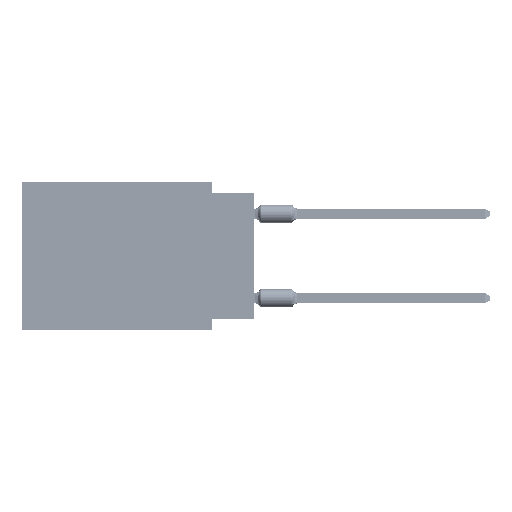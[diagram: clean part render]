
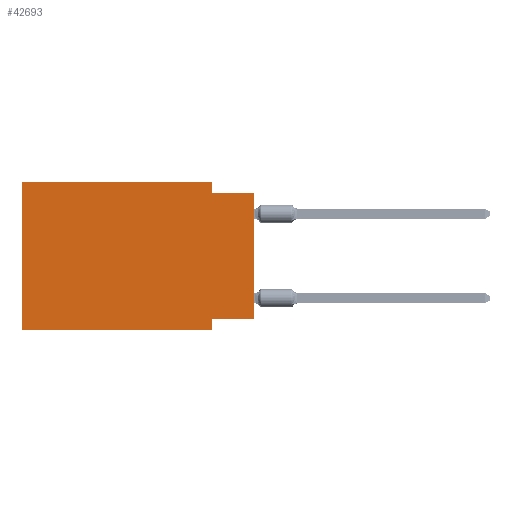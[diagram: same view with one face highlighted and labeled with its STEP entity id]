
A CAD part, left-side view. The second image highlights one B-rep face of the part: STEP entity #42693.
In plain terms, the highlighted planar face has unit normal (-1, 0, 0).
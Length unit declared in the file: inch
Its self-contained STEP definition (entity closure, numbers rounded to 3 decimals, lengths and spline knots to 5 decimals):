
#1951 = EDGE_CURVE ( 'NONE', #13070, #85493, #46114, .T. ) ;
#2984 = VECTOR ( 'NONE', #79374, 39.37008 ) ;
#6643 = DIRECTION ( 'NONE',  ( 0., 0., -1. ) ) ;
#12894 = LINE ( 'NONE', #95764, #94227 ) ;
#13070 = VERTEX_POINT ( 'NONE', #76382 ) ;
#13754 = VERTEX_POINT ( 'NONE', #31894 ) ;
#15573 = EDGE_CURVE ( 'NONE', #13754, #57237, #38477, .T. ) ;
#16626 = ORIENTED_EDGE ( 'NONE', *, *, #24717, .F. ) ;
#17068 = VECTOR ( 'NONE', #44980, 39.37008 ) ;
#18312 = CARTESIAN_POINT ( 'NONE',  ( 0., 0.55, 0. ) ) ;
#18451 = EDGE_LOOP ( 'NONE', ( #107226, #99488, #53369, #82596, #94950, #79710, #16626, #52889 ) ) ;
#20649 = CARTESIAN_POINT ( 'NONE',  ( 0., 0., 0. ) ) ;
#21079 = DIRECTION ( 'NONE',  ( 0., 0., -1. ) ) ;
#23228 = AXIS2_PLACEMENT_3D ( 'NONE', #80891, #97754, #73250 ) ;
#24717 = EDGE_CURVE ( 'NONE', #39532, #85493, #71554, .T. ) ;
#27841 = VECTOR ( 'NONE', #30315, 39.37008 ) ;
#30103 = VERTEX_POINT ( 'NONE', #82910 ) ;
#30315 = DIRECTION ( 'NONE',  ( 0., 0., 1. ) ) ;
#30742 = LINE ( 'NONE', #63977, #17068 ) ;
#31894 = CARTESIAN_POINT ( 'NONE',  ( 0., 0.1, -0.025 ) ) ;
#32446 = CARTESIAN_POINT ( 'NONE',  ( 0., 0.55, 0. ) ) ;
#36902 = LINE ( 'NONE', #86508, #27841 ) ;
#38477 = LINE ( 'NONE', #103917, #2984 ) ;
#39463 = PLANE ( 'NONE',  #23228 ) ;
#39532 = VERTEX_POINT ( 'NONE', #76016 ) ;
#42693 = ADVANCED_FACE ( 'NONE', ( #46021 ), #39463, .F. ) ;
#44980 = DIRECTION ( 'NONE',  ( 0., 1., 0. ) ) ;
#46021 = FACE_OUTER_BOUND ( 'NONE', #18451, .T. ) ;
#46114 = LINE ( 'NONE', #80439, #86129 ) ;
#49419 = VECTOR ( 'NONE', #6643, 39.37008 ) ;
#52889 = ORIENTED_EDGE ( 'NONE', *, *, #91686, .F. ) ;
#53369 = ORIENTED_EDGE ( 'NONE', *, *, #80028, .F. ) ;
#53909 = DIRECTION ( 'NONE',  ( 0., 0., 1. ) ) ;
#55893 = DIRECTION ( 'NONE',  ( 0., -1., 0. ) ) ;
#56287 = VECTOR ( 'NONE', #84206, 39.37008 ) ;
#57237 = VERTEX_POINT ( 'NONE', #66730 ) ;
#63977 = CARTESIAN_POINT ( 'NONE',  ( 0., 0., -0.325 ) ) ;
#66730 = CARTESIAN_POINT ( 'NONE',  ( 0., 0., -0.025 ) ) ;
#71554 = LINE ( 'NONE', #72632, #49419 ) ;
#72632 = CARTESIAN_POINT ( 'NONE',  ( 0., 0.1, -0.35 ) ) ;
#73250 = DIRECTION ( 'NONE',  ( 0., 0., -1. ) ) ;
#74839 = EDGE_CURVE ( 'NONE', #81567, #102932, #107123, .T. ) ;
#76016 = CARTESIAN_POINT ( 'NONE',  ( 0., 0.1, -0.325 ) ) ;
#76246 = VECTOR ( 'NONE', #53909, 39.37008 ) ;
#76382 = CARTESIAN_POINT ( 'NONE',  ( 0., 0.55, -0.35 ) ) ;
#79374 = DIRECTION ( 'NONE',  ( 0., -1., 0. ) ) ;
#79710 = ORIENTED_EDGE ( 'NONE', *, *, #1951, .T. ) ;
#80028 = EDGE_CURVE ( 'NONE', #102932, #13754, #12894, .T. ) ;
#80439 = CARTESIAN_POINT ( 'NONE',  ( 0., 0.55, -0.35 ) ) ;
#80891 = CARTESIAN_POINT ( 'NONE',  ( 0., 0.55, 0. ) ) ;
#81567 = VERTEX_POINT ( 'NONE', #18312 ) ;
#82596 = ORIENTED_EDGE ( 'NONE', *, *, #74839, .F. ) ;
#82910 = CARTESIAN_POINT ( 'NONE',  ( 0., 0., -0.325 ) ) ;
#84206 = DIRECTION ( 'NONE',  ( 0., -1., 0. ) ) ;
#84910 = CARTESIAN_POINT ( 'NONE',  ( 0., 0.1, 0. ) ) ;
#85493 = VERTEX_POINT ( 'NONE', #92597 ) ;
#86129 = VECTOR ( 'NONE', #55893, 39.37008 ) ;
#86508 = CARTESIAN_POINT ( 'NONE',  ( 0., 0.55, 0. ) ) ;
#91686 = EDGE_CURVE ( 'NONE', #30103, #39532, #30742, .T. ) ;
#92597 = CARTESIAN_POINT ( 'NONE',  ( 0., 0.1, -0.35 ) ) ;
#94227 = VECTOR ( 'NONE', #21079, 39.37008 ) ;
#94950 = ORIENTED_EDGE ( 'NONE', *, *, #103175, .F. ) ;
#95764 = CARTESIAN_POINT ( 'NONE',  ( 0., 0.1, 0. ) ) ;
#97754 = DIRECTION ( 'NONE',  ( 1., 0., 0. ) ) ;
#99245 = EDGE_CURVE ( 'NONE', #30103, #57237, #101391, .T. ) ;
#99488 = ORIENTED_EDGE ( 'NONE', *, *, #15573, .F. ) ;
#101391 = LINE ( 'NONE', #20649, #76246 ) ;
#102932 = VERTEX_POINT ( 'NONE', #84910 ) ;
#103175 = EDGE_CURVE ( 'NONE', #13070, #81567, #36902, .T. ) ;
#103917 = CARTESIAN_POINT ( 'NONE',  ( 0., 0., -0.025 ) ) ;
#107123 = LINE ( 'NONE', #32446, #56287 ) ;
#107226 = ORIENTED_EDGE ( 'NONE', *, *, #99245, .T. ) ;
